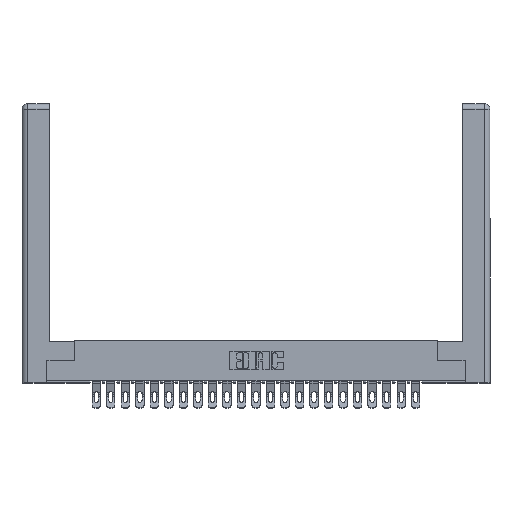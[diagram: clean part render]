
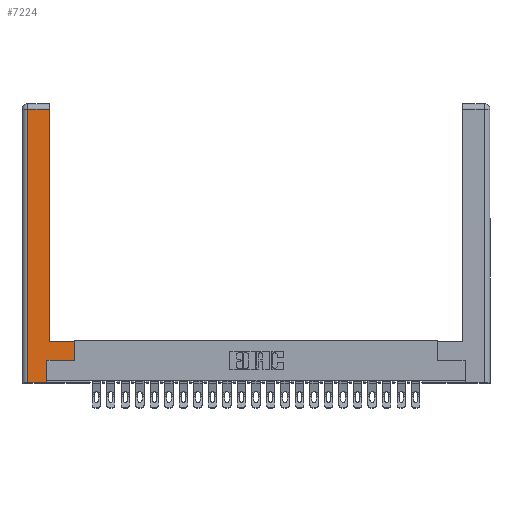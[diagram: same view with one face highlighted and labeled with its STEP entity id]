
A CAD part, top view. The second image highlights one B-rep face of the part: STEP entity #7224.
In plain terms, the highlighted planar face has unit normal (0, 0, 1).
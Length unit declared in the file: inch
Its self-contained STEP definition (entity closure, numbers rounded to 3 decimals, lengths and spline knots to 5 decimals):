
#466 = VERTEX_POINT ( 'NONE', #22937 ) ;
#823 = CARTESIAN_POINT ( 'NONE',  ( 0.295, 0.45, 0. ) ) ;
#1308 = EDGE_CURVE ( 'NONE', #28294, #21624, #26865, .T. ) ;
#2368 = LINE ( 'NONE', #15666, #18969 ) ;
#3729 = DIRECTION ( 'NONE',  ( 0., 1., 0. ) ) ;
#4203 = CARTESIAN_POINT ( 'NONE',  ( 0.265, 0., 0. ) ) ;
#4547 = EDGE_CURVE ( 'NONE', #23620, #13303, #20911, .T. ) ;
#4632 = LINE ( 'NONE', #18514, #17051 ) ;
#4774 = VECTOR ( 'NONE', #6447, 39.37008 ) ;
#5431 = ORIENTED_EDGE ( 'NONE', *, *, #24986, .T. ) ;
#6118 = EDGE_CURVE ( 'NONE', #13303, #466, #4632, .T. ) ;
#6126 = ORIENTED_EDGE ( 'NONE', *, *, #12093, .T. ) ;
#6447 = DIRECTION ( 'NONE',  ( 1., 0., 0. ) ) ;
#7224 = ADVANCED_FACE ( 'NONE', ( #14555 ), #9751, .F. ) ;
#8808 = ORIENTED_EDGE ( 'NONE', *, *, #17610, .T. ) ;
#8816 = DIRECTION ( 'NONE',  ( -1., 0., 0. ) ) ;
#9526 = CARTESIAN_POINT ( 'NONE',  ( 0.565, 0.245, 0. ) ) ;
#9751 = PLANE ( 'NONE',  #27239 ) ;
#9885 = VECTOR ( 'NONE', #28891, 39.37008 ) ;
#10128 = CARTESIAN_POINT ( 'NONE',  ( 0.565, 0.245, 0. ) ) ;
#10229 = DIRECTION ( 'NONE',  ( 0., 1., 0. ) ) ;
#10320 = CARTESIAN_POINT ( 'NONE',  ( 0.265, 0., 0. ) ) ;
#11112 = VERTEX_POINT ( 'NONE', #21340 ) ;
#12093 = EDGE_CURVE ( 'NONE', #23552, #11112, #25362, .T. ) ;
#12376 = EDGE_LOOP ( 'NONE', ( #21887, #30004, #24306, #5431, #6126, #8808, #25448, #13844 ) ) ;
#12525 = CARTESIAN_POINT ( 'NONE',  ( 0.295, 3., 0. ) ) ;
#12569 = CARTESIAN_POINT ( 'NONE',  ( 0.265, 0.245, 0. ) ) ;
#12625 = LINE ( 'NONE', #9526, #29544 ) ;
#13303 = VERTEX_POINT ( 'NONE', #28564 ) ;
#13844 = ORIENTED_EDGE ( 'NONE', *, *, #1308, .T. ) ;
#14555 = FACE_OUTER_BOUND ( 'NONE', #12376, .T. ) ;
#15494 = DIRECTION ( 'NONE',  ( -1., 0., 0. ) ) ;
#15666 = CARTESIAN_POINT ( 'NONE',  ( 0.565, 0.45, 0. ) ) ;
#16539 = LINE ( 'NONE', #12525, #28279 ) ;
#16877 = CARTESIAN_POINT ( 'NONE',  ( 0., 0., 0. ) ) ;
#17051 = VECTOR ( 'NONE', #18307, 39.37008 ) ;
#17610 = EDGE_CURVE ( 'NONE', #11112, #26791, #12625, .T. ) ;
#18307 = DIRECTION ( 'NONE',  ( 0., -1., 0. ) ) ;
#18514 = CARTESIAN_POINT ( 'NONE',  ( 0.0615, 0., 0. ) ) ;
#18969 = VECTOR ( 'NONE', #3729, 39.37008 ) ;
#19101 = CARTESIAN_POINT ( 'NONE',  ( 0.565, 0.45, 0. ) ) ;
#20242 = CARTESIAN_POINT ( 'NONE',  ( 0.0615, 2.94, 0. ) ) ;
#20593 = CARTESIAN_POINT ( 'NONE',  ( 0.295, 0.45, 0. ) ) ;
#20656 = LINE ( 'NONE', #4203, #4774 ) ;
#20911 = LINE ( 'NONE', #20242, #26747 ) ;
#21340 = CARTESIAN_POINT ( 'NONE',  ( 0.265, 0.245, 0. ) ) ;
#21624 = VERTEX_POINT ( 'NONE', #823 ) ;
#21887 = ORIENTED_EDGE ( 'NONE', *, *, #25482, .T. ) ;
#22829 = VECTOR ( 'NONE', #8816, 39.37008 ) ;
#22937 = CARTESIAN_POINT ( 'NONE',  ( 0.0615, 0., 0. ) ) ;
#23552 = VERTEX_POINT ( 'NONE', #10320 ) ;
#23620 = VERTEX_POINT ( 'NONE', #24627 ) ;
#23950 = DIRECTION ( 'NONE',  ( -1., 0., 0. ) ) ;
#24306 = ORIENTED_EDGE ( 'NONE', *, *, #6118, .T. ) ;
#24627 = CARTESIAN_POINT ( 'NONE',  ( 0.295, 2.94, 0. ) ) ;
#24986 = EDGE_CURVE ( 'NONE', #466, #23552, #20656, .T. ) ;
#25362 = LINE ( 'NONE', #12569, #9885 ) ;
#25448 = ORIENTED_EDGE ( 'NONE', *, *, #29982, .T. ) ;
#25482 = EDGE_CURVE ( 'NONE', #21624, #23620, #16539, .T. ) ;
#25595 = DIRECTION ( 'NONE',  ( 1., 0., 0. ) ) ;
#26747 = VECTOR ( 'NONE', #15494, 39.37008 ) ;
#26791 = VERTEX_POINT ( 'NONE', #10128 ) ;
#26865 = LINE ( 'NONE', #20593, #22829 ) ;
#27239 = AXIS2_PLACEMENT_3D ( 'NONE', #16877, #28266, #23950 ) ;
#28266 = DIRECTION ( 'NONE',  ( 0., 0., -1. ) ) ;
#28279 = VECTOR ( 'NONE', #10229, 39.37008 ) ;
#28294 = VERTEX_POINT ( 'NONE', #19101 ) ;
#28564 = CARTESIAN_POINT ( 'NONE',  ( 0.0615, 2.94, 0. ) ) ;
#28891 = DIRECTION ( 'NONE',  ( 0., 1., 0. ) ) ;
#29544 = VECTOR ( 'NONE', #25595, 39.37008 ) ;
#29982 = EDGE_CURVE ( 'NONE', #26791, #28294, #2368, .T. ) ;
#30004 = ORIENTED_EDGE ( 'NONE', *, *, #4547, .T. ) ;
